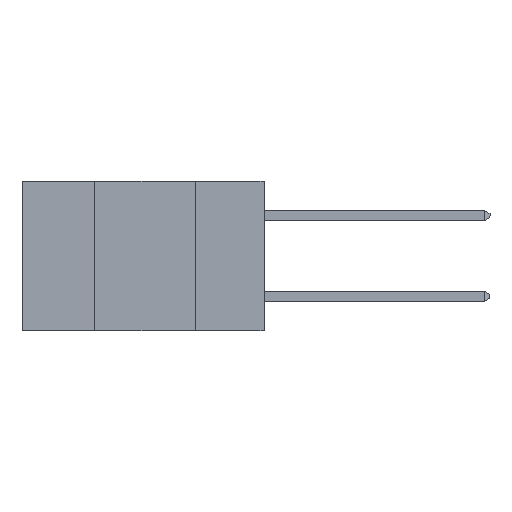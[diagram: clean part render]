
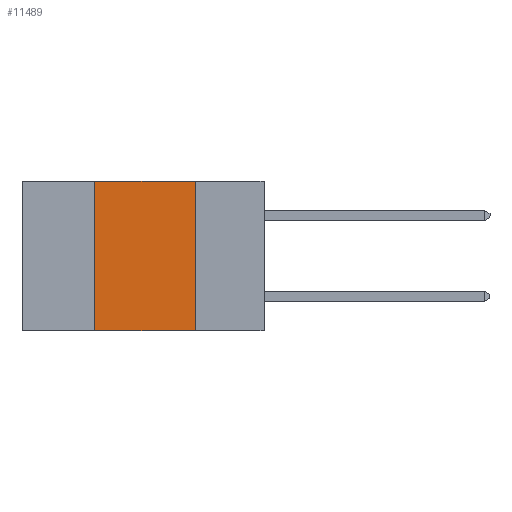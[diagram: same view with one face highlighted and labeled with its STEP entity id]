
A CAD part, left-side view. The second image highlights one B-rep face of the part: STEP entity #11489.
In plain terms, the highlighted planar face has unit normal (-1, 0, 0).
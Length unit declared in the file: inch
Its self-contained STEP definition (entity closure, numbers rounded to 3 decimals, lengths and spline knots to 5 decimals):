
#119 = CARTESIAN_POINT ( 'NONE',  ( 0., 0.17, 0. ) ) ;
#214 = DIRECTION ( 'NONE',  ( 0., -1., 0. ) ) ;
#333 = CARTESIAN_POINT ( 'NONE',  ( 0., 0.42, 0. ) ) ;
#863 = DIRECTION ( 'NONE',  ( 1., 0., 0. ) ) ;
#1799 = VERTEX_POINT ( 'NONE', #333 ) ;
#1986 = VECTOR ( 'NONE', #21924, 39.37008 ) ;
#2435 = VECTOR ( 'NONE', #16598, 39.37008 ) ;
#2955 = VECTOR ( 'NONE', #214, 39.37008 ) ;
#3292 = EDGE_CURVE ( 'NONE', #18524, #17169, #6544, .T. ) ;
#3445 = EDGE_CURVE ( 'NONE', #1799, #18524, #3857, .T. ) ;
#3476 = EDGE_LOOP ( 'NONE', ( #8315, #13890, #7002, #18615 ) ) ;
#3857 = LINE ( 'NONE', #21505, #12528 ) ;
#4808 = VERTEX_POINT ( 'NONE', #20559 ) ;
#5299 = AXIS2_PLACEMENT_3D ( 'NONE', #9474, #863, #13011 ) ;
#5374 = CARTESIAN_POINT ( 'NONE',  ( 0., 0.6, -0.37 ) ) ;
#6544 = LINE ( 'NONE', #22032, #1986 ) ;
#7002 = ORIENTED_EDGE ( 'NONE', *, *, #21134, .F. ) ;
#7558 = FACE_OUTER_BOUND ( 'NONE', #3476, .T. ) ;
#8315 = ORIENTED_EDGE ( 'NONE', *, *, #3292, .F. ) ;
#9474 = CARTESIAN_POINT ( 'NONE',  ( 0., 0.6, 0. ) ) ;
#11489 = ADVANCED_FACE ( 'NONE', ( #7558 ), #21603, .F. ) ;
#11916 = CARTESIAN_POINT ( 'NONE',  ( 0., 0.17, -0.37 ) ) ;
#12528 = VECTOR ( 'NONE', #21452, 39.37008 ) ;
#13011 = DIRECTION ( 'NONE',  ( 0., 0., -1. ) ) ;
#13890 = ORIENTED_EDGE ( 'NONE', *, *, #3445, .F. ) ;
#15799 = LINE ( 'NONE', #21739, #2435 ) ;
#16598 = DIRECTION ( 'NONE',  ( 0., 0., 1. ) ) ;
#17169 = VERTEX_POINT ( 'NONE', #11916 ) ;
#17899 = LINE ( 'NONE', #5374, #2955 ) ;
#18524 = VERTEX_POINT ( 'NONE', #119 ) ;
#18615 = ORIENTED_EDGE ( 'NONE', *, *, #21548, .T. ) ;
#20559 = CARTESIAN_POINT ( 'NONE',  ( 0., 0.42, -0.37 ) ) ;
#21134 = EDGE_CURVE ( 'NONE', #4808, #1799, #15799, .T. ) ;
#21452 = DIRECTION ( 'NONE',  ( 0., -1., 0. ) ) ;
#21505 = CARTESIAN_POINT ( 'NONE',  ( 0., 0.6, 0. ) ) ;
#21548 = EDGE_CURVE ( 'NONE', #4808, #17169, #17899, .T. ) ;
#21603 = PLANE ( 'NONE',  #5299 ) ;
#21739 = CARTESIAN_POINT ( 'NONE',  ( 0., 0.42, 0. ) ) ;
#21924 = DIRECTION ( 'NONE',  ( 0., 0., -1. ) ) ;
#22032 = CARTESIAN_POINT ( 'NONE',  ( 0., 0.17, 0. ) ) ;
